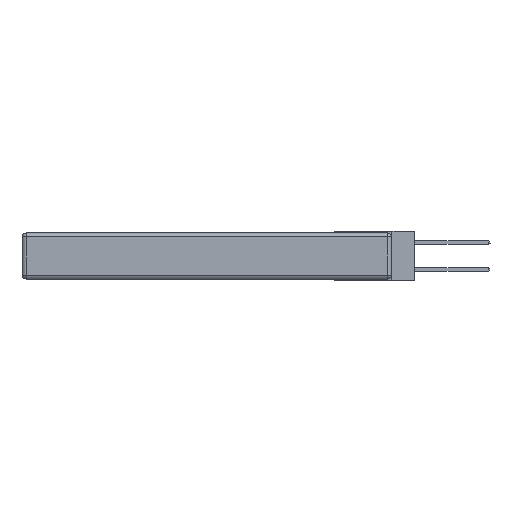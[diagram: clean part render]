
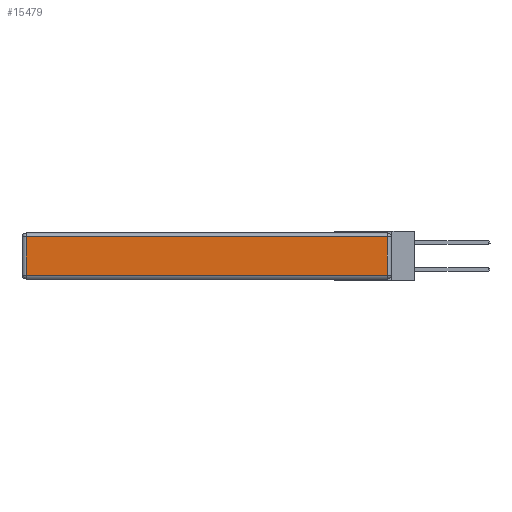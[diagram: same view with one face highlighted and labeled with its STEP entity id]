
A CAD part, left-side view. The second image highlights one B-rep face of the part: STEP entity #15479.
In plain terms, the highlighted planar face has unit normal (-1, 0, 0).
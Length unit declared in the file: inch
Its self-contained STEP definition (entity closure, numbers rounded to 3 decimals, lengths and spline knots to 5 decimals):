
#796 = CARTESIAN_POINT ( 'NONE',  ( 0., 0.03, -0.343 ) ) ;
#1124 = VERTEX_POINT ( 'NONE', #15663 ) ;
#1339 = CARTESIAN_POINT ( 'NONE',  ( 0., 0., -0.343 ) ) ;
#1899 = DIRECTION ( 'NONE',  ( 0., -1., 0. ) ) ;
#2123 = LINE ( 'NONE', #796, #15010 ) ;
#2332 = DIRECTION ( 'NONE',  ( 0., 0., 1. ) ) ;
#2486 = CARTESIAN_POINT ( 'NONE',  ( 0., 2.72, -0.313 ) ) ;
#2639 = DIRECTION ( 'NONE',  ( 0., 1., 0. ) ) ;
#3407 = CARTESIAN_POINT ( 'NONE',  ( 0., 0., -0.313 ) ) ;
#3500 = VERTEX_POINT ( 'NONE', #2486 ) ;
#3555 = EDGE_LOOP ( 'NONE', ( #12748, #7516, #17508, #15882 ) ) ;
#3638 = VERTEX_POINT ( 'NONE', #18096 ) ;
#3783 = CARTESIAN_POINT ( 'NONE',  ( 0., 2.72, -0.343 ) ) ;
#5283 = DIRECTION ( 'NONE',  ( 0., 0., -1. ) ) ;
#5665 = CARTESIAN_POINT ( 'NONE',  ( 0., 2.75, -0.03 ) ) ;
#5751 = LINE ( 'NONE', #3407, #9235 ) ;
#6630 = EDGE_CURVE ( 'NONE', #13219, #1124, #2123, .T. ) ;
#7359 = DIRECTION ( 'NONE',  ( 0., 0., 1. ) ) ;
#7516 = ORIENTED_EDGE ( 'NONE', *, *, #6630, .T. ) ;
#9235 = VECTOR ( 'NONE', #1899, 39.37008 ) ;
#9810 = VECTOR ( 'NONE', #2639, 39.37008 ) ;
#10161 = PLANE ( 'NONE',  #10332 ) ;
#10332 = AXIS2_PLACEMENT_3D ( 'NONE', #1339, #11678, #7359 ) ;
#10882 = LINE ( 'NONE', #3783, #13230 ) ;
#11374 = FACE_OUTER_BOUND ( 'NONE', #3555, .T. ) ;
#11678 = DIRECTION ( 'NONE',  ( -1., 0., 0. ) ) ;
#12748 = ORIENTED_EDGE ( 'NONE', *, *, #16355, .T. ) ;
#13219 = VERTEX_POINT ( 'NONE', #16003 ) ;
#13230 = VECTOR ( 'NONE', #5283, 39.37008 ) ;
#14283 = LINE ( 'NONE', #5665, #9810 ) ;
#15010 = VECTOR ( 'NONE', #2332, 39.37008 ) ;
#15479 = ADVANCED_FACE ( 'NONE', ( #11374 ), #10161, .T. ) ;
#15663 = CARTESIAN_POINT ( 'NONE',  ( 0., 0.03, -0.03 ) ) ;
#15796 = EDGE_CURVE ( 'NONE', #3638, #3500, #10882, .T. ) ;
#15882 = ORIENTED_EDGE ( 'NONE', *, *, #15796, .T. ) ;
#16003 = CARTESIAN_POINT ( 'NONE',  ( 0., 0.03, -0.313 ) ) ;
#16355 = EDGE_CURVE ( 'NONE', #3500, #13219, #5751, .T. ) ;
#17508 = ORIENTED_EDGE ( 'NONE', *, *, #18589, .T. ) ;
#18096 = CARTESIAN_POINT ( 'NONE',  ( 0., 2.72, -0.03 ) ) ;
#18589 = EDGE_CURVE ( 'NONE', #1124, #3638, #14283, .T. ) ;
